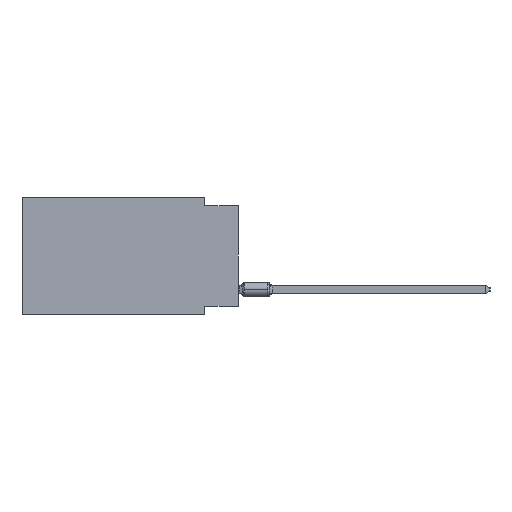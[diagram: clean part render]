
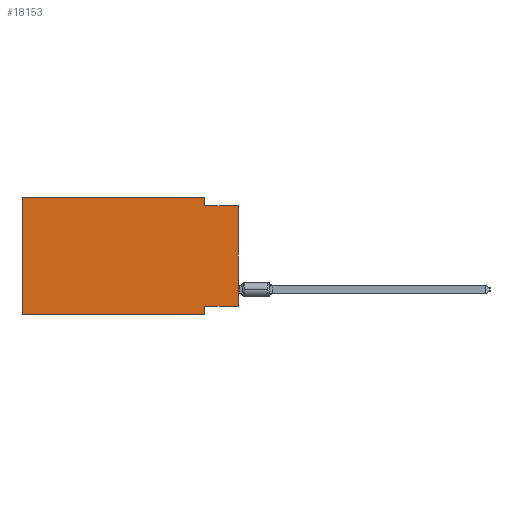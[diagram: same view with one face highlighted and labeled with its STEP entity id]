
A CAD part, left-side view. The second image highlights one B-rep face of the part: STEP entity #18153.
In plain terms, the highlighted planar face has unit normal (-1, 0, 0).
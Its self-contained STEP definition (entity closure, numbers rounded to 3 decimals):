
#88 = CARTESIAN_POINT ( 'NONE',  ( 0., 2.54, 0. ) ) ;
#1051 = VECTOR ( 'NONE', #9977, 1000. ) ;
#1545 = ORIENTED_EDGE ( 'NONE', *, *, #18907, .T. ) ;
#2013 = CARTESIAN_POINT ( 'NONE',  ( 0., 0., -8.255 ) ) ;
#2116 = ORIENTED_EDGE ( 'NONE', *, *, #5497, .F. ) ;
#2246 = CARTESIAN_POINT ( 'NONE',  ( 0., 16.383, 0. ) ) ;
#2329 = CARTESIAN_POINT ( 'NONE',  ( 0., 0., 0. ) ) ;
#2567 = PLANE ( 'NONE',  #20942 ) ;
#3045 = DIRECTION ( 'NONE',  ( 0., 0., -1. ) ) ;
#3281 = CARTESIAN_POINT ( 'NONE',  ( 0., 16.383, 0. ) ) ;
#3671 = LINE ( 'NONE', #28130, #28108 ) ;
#4311 = CARTESIAN_POINT ( 'NONE',  ( 0., 16.383, -8.89 ) ) ;
#4616 = CARTESIAN_POINT ( 'NONE',  ( 0., 16.383, -8.89 ) ) ;
#4823 = VECTOR ( 'NONE', #28781, 1000. ) ;
#5497 = EDGE_CURVE ( 'NONE', #31224, #28512, #9025, .T. ) ;
#5635 = EDGE_CURVE ( 'NONE', #13069, #22650, #16812, .T. ) ;
#5708 = ORIENTED_EDGE ( 'NONE', *, *, #14270, .F. ) ;
#6027 = CARTESIAN_POINT ( 'NONE',  ( 0., 0., -0.635 ) ) ;
#6106 = EDGE_CURVE ( 'NONE', #28512, #25919, #3671, .T. ) ;
#6132 = EDGE_LOOP ( 'NONE', ( #1545, #21362, #10723, #29514, #2116, #14843, #22756, #5708 ) ) ;
#6695 = LINE ( 'NONE', #2013, #25647 ) ;
#6853 = DIRECTION ( 'NONE',  ( 0., 1., 0. ) ) ;
#6926 = DIRECTION ( 'NONE',  ( 0., -1., 0. ) ) ;
#7033 = VECTOR ( 'NONE', #27410, 1000. ) ;
#7623 = CARTESIAN_POINT ( 'NONE',  ( 0., 2.54, 0. ) ) ;
#9025 = LINE ( 'NONE', #11304, #4823 ) ;
#9199 = CARTESIAN_POINT ( 'NONE',  ( 0., 2.54, -8.255 ) ) ;
#9639 = LINE ( 'NONE', #4616, #27833 ) ;
#9977 = DIRECTION ( 'NONE',  ( 0., 0., -1. ) ) ;
#10163 = CARTESIAN_POINT ( 'NONE',  ( 0., 0., -8.255 ) ) ;
#10723 = ORIENTED_EDGE ( 'NONE', *, *, #31377, .F. ) ;
#11304 = CARTESIAN_POINT ( 'NONE',  ( 0., 16.383, 0. ) ) ;
#12285 = DIRECTION ( 'NONE',  ( 0., 0., -1. ) ) ;
#13069 = VERTEX_POINT ( 'NONE', #21967 ) ;
#13135 = VECTOR ( 'NONE', #3045, 1000. ) ;
#14026 = VERTEX_POINT ( 'NONE', #10163 ) ;
#14270 = EDGE_CURVE ( 'NONE', #14026, #17989, #6695, .T. ) ;
#14711 = DIRECTION ( 'NONE',  ( 1., 0., 0. ) ) ;
#14843 = ORIENTED_EDGE ( 'NONE', *, *, #20884, .T. ) ;
#14863 = CARTESIAN_POINT ( 'NONE',  ( 0., 0., -0.635 ) ) ;
#16812 = LINE ( 'NONE', #14863, #31197 ) ;
#17066 = LINE ( 'NONE', #2329, #7033 ) ;
#17309 = CARTESIAN_POINT ( 'NONE',  ( 0., 2.54, -8.89 ) ) ;
#17989 = VERTEX_POINT ( 'NONE', #9199 ) ;
#18153 = ADVANCED_FACE ( 'NONE', ( #24428 ), #2567, .F. ) ;
#18416 = DIRECTION ( 'NONE',  ( 0., -1., 0. ) ) ;
#18907 = EDGE_CURVE ( 'NONE', #14026, #22650, #17066, .T. ) ;
#19196 = DIRECTION ( 'NONE',  ( 0., -1., 0. ) ) ;
#20884 = EDGE_CURVE ( 'NONE', #31224, #21850, #9639, .T. ) ;
#20942 = AXIS2_PLACEMENT_3D ( 'NONE', #2246, #14711, #12285 ) ;
#21362 = ORIENTED_EDGE ( 'NONE', *, *, #5635, .F. ) ;
#21850 = VERTEX_POINT ( 'NONE', #28128 ) ;
#21967 = CARTESIAN_POINT ( 'NONE',  ( 0., 2.54, -0.635 ) ) ;
#22275 = LINE ( 'NONE', #88, #1051 ) ;
#22650 = VERTEX_POINT ( 'NONE', #6027 ) ;
#22756 = ORIENTED_EDGE ( 'NONE', *, *, #26272, .F. ) ;
#22957 = LINE ( 'NONE', #17309, #13135 ) ;
#24428 = FACE_OUTER_BOUND ( 'NONE', #6132, .T. ) ;
#25647 = VECTOR ( 'NONE', #6853, 1000. ) ;
#25919 = VERTEX_POINT ( 'NONE', #7623 ) ;
#26272 = EDGE_CURVE ( 'NONE', #17989, #21850, #22957, .T. ) ;
#27410 = DIRECTION ( 'NONE',  ( 0., 0., 1. ) ) ;
#27833 = VECTOR ( 'NONE', #19196, 1000. ) ;
#28108 = VECTOR ( 'NONE', #18416, 1000. ) ;
#28128 = CARTESIAN_POINT ( 'NONE',  ( 0., 2.54, -8.89 ) ) ;
#28130 = CARTESIAN_POINT ( 'NONE',  ( 0., 16.383, 0. ) ) ;
#28512 = VERTEX_POINT ( 'NONE', #3281 ) ;
#28781 = DIRECTION ( 'NONE',  ( 0., 0., 1. ) ) ;
#29514 = ORIENTED_EDGE ( 'NONE', *, *, #6106, .F. ) ;
#31197 = VECTOR ( 'NONE', #6926, 1000. ) ;
#31224 = VERTEX_POINT ( 'NONE', #4311 ) ;
#31377 = EDGE_CURVE ( 'NONE', #25919, #13069, #22275, .T. ) ;
